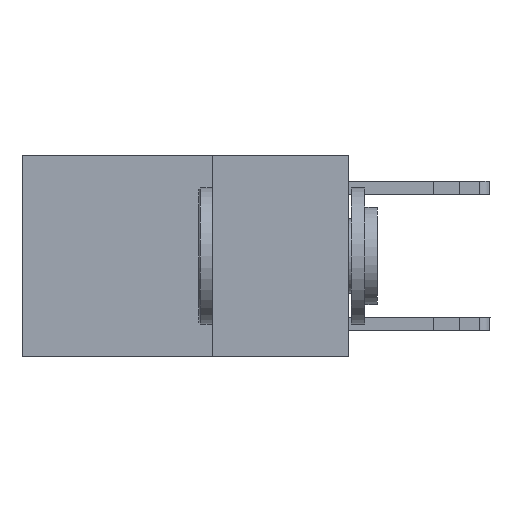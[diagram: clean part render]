
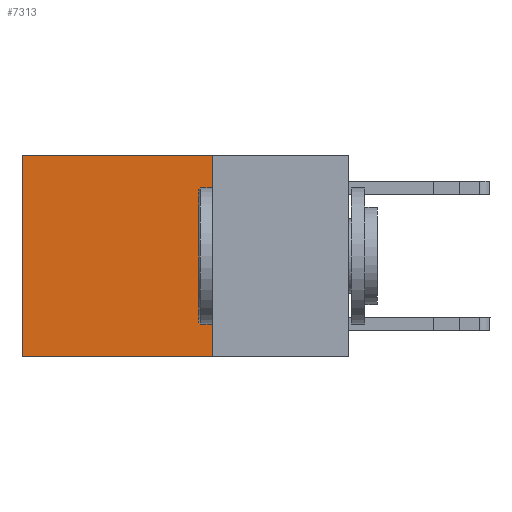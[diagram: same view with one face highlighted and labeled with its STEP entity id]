
A CAD part, left-side view. The second image highlights one B-rep face of the part: STEP entity #7313.
In plain terms, the highlighted planar face has unit normal (-1, 0, 0).
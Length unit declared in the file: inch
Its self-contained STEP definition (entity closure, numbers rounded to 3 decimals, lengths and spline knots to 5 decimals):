
#1038 = ORIENTED_EDGE ( 'NONE', *, *, #5639, .F. ) ;
#1094 = CARTESIAN_POINT ( 'NONE',  ( 0.2625, 0.25, 0. ) ) ;
#1115 = LINE ( 'NONE', #14150, #3394 ) ;
#1159 = DIRECTION ( 'NONE',  ( 0., 0., -1. ) ) ;
#1621 = ORIENTED_EDGE ( 'NONE', *, *, #13781, .T. ) ;
#2578 = CARTESIAN_POINT ( 'NONE',  ( 0.2625, 0.25, 0. ) ) ;
#3128 = CARTESIAN_POINT ( 'NONE',  ( 0.2625, 0.25, -0.37 ) ) ;
#3394 = VECTOR ( 'NONE', #7633, 39.37008 ) ;
#3625 = VERTEX_POINT ( 'NONE', #8207 ) ;
#4822 = DIRECTION ( 'NONE',  ( 0., 1., 0. ) ) ;
#5267 = DIRECTION ( 'NONE',  ( 1., 0., 0. ) ) ;
#5639 = EDGE_CURVE ( 'NONE', #6068, #16597, #8698, .T. ) ;
#6068 = VERTEX_POINT ( 'NONE', #7838 ) ;
#6526 = LINE ( 'NONE', #11785, #11522 ) ;
#7139 = EDGE_LOOP ( 'NONE', ( #12764, #13932, #1038, #1621 ) ) ;
#7313 = ADVANCED_FACE ( 'NONE', ( #10615 ), #9172, .F. ) ;
#7633 = DIRECTION ( 'NONE',  ( 0., 1., 0. ) ) ;
#7760 = VECTOR ( 'NONE', #4822, 39.37008 ) ;
#7798 = VERTEX_POINT ( 'NONE', #15613 ) ;
#7838 = CARTESIAN_POINT ( 'NONE',  ( 0.2625, 0.25, 0. ) ) ;
#8207 = CARTESIAN_POINT ( 'NONE',  ( 0.2625, 0.6, -0.37 ) ) ;
#8628 = VECTOR ( 'NONE', #9040, 39.37008 ) ;
#8698 = LINE ( 'NONE', #11264, #8628 ) ;
#9040 = DIRECTION ( 'NONE',  ( 0., 0., -1. ) ) ;
#9172 = PLANE ( 'NONE',  #12275 ) ;
#9526 = EDGE_CURVE ( 'NONE', #7798, #3625, #6526, .T. ) ;
#10529 = DIRECTION ( 'NONE',  ( 0., 0., -1. ) ) ;
#10615 = FACE_OUTER_BOUND ( 'NONE', #7139, .T. ) ;
#11264 = CARTESIAN_POINT ( 'NONE',  ( 0.2625, 0.25, 0. ) ) ;
#11290 = LINE ( 'NONE', #1094, #7760 ) ;
#11522 = VECTOR ( 'NONE', #1159, 39.37008 ) ;
#11785 = CARTESIAN_POINT ( 'NONE',  ( 0.2625, 0.6, 0. ) ) ;
#12275 = AXIS2_PLACEMENT_3D ( 'NONE', #2578, #5267, #10529 ) ;
#12764 = ORIENTED_EDGE ( 'NONE', *, *, #9526, .T. ) ;
#13781 = EDGE_CURVE ( 'NONE', #6068, #7798, #11290, .T. ) ;
#13932 = ORIENTED_EDGE ( 'NONE', *, *, #16757, .F. ) ;
#14150 = CARTESIAN_POINT ( 'NONE',  ( 0.2625, 0.25, -0.37 ) ) ;
#15613 = CARTESIAN_POINT ( 'NONE',  ( 0.2625, 0.6, 0. ) ) ;
#16597 = VERTEX_POINT ( 'NONE', #3128 ) ;
#16757 = EDGE_CURVE ( 'NONE', #16597, #3625, #1115, .T. ) ;
